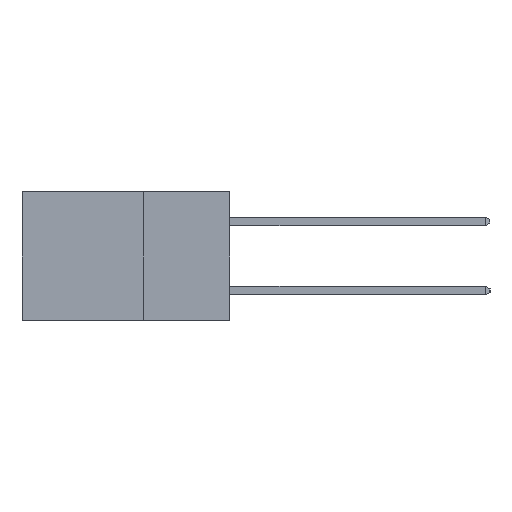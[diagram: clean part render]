
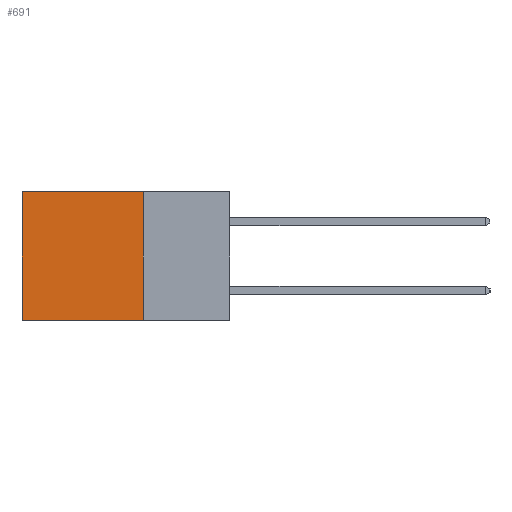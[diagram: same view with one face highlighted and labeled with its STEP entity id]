
A CAD part, left-side view. The second image highlights one B-rep face of the part: STEP entity #691.
In plain terms, the highlighted planar face has unit normal (-1, 0, 0).
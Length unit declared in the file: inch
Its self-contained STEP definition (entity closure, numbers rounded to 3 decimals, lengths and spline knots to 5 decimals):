
#233 = VECTOR ( 'NONE', #857, 39.37008 ) ;
#343 = DIRECTION ( 'NONE',  ( 0., 0., -1. ) ) ;
#485 = AXIS2_PLACEMENT_3D ( 'NONE', #15992, #3323, #12492 ) ;
#618 = ORIENTED_EDGE ( 'NONE', *, *, #6132, .F. ) ;
#691 = ADVANCED_FACE ( 'NONE', ( #9687 ), #2797, .F. ) ;
#857 = DIRECTION ( 'NONE',  ( 0., 1., 0. ) ) ;
#2797 = PLANE ( 'NONE',  #485 ) ;
#2810 = VERTEX_POINT ( 'NONE', #12886 ) ;
#3323 = DIRECTION ( 'NONE',  ( 1., 0., 0. ) ) ;
#3816 = EDGE_LOOP ( 'NONE', ( #7078, #16135, #618, #5748 ) ) ;
#4858 = DIRECTION ( 'NONE',  ( 0., 0., -1. ) ) ;
#4925 = VERTEX_POINT ( 'NONE', #6844 ) ;
#5748 = ORIENTED_EDGE ( 'NONE', *, *, #8540, .T. ) ;
#6132 = EDGE_CURVE ( 'NONE', #9060, #4925, #10364, .T. ) ;
#6844 = CARTESIAN_POINT ( 'NONE',  ( 0.2615, 0.25, -0.37 ) ) ;
#7078 = ORIENTED_EDGE ( 'NONE', *, *, #8276, .T. ) ;
#7464 = CARTESIAN_POINT ( 'NONE',  ( 0.2615, 0.25, -0.37 ) ) ;
#8150 = LINE ( 'NONE', #7464, #12602 ) ;
#8276 = EDGE_CURVE ( 'NONE', #2810, #11419, #8672, .T. ) ;
#8512 = CARTESIAN_POINT ( 'NONE',  ( 0.2615, 0.25, 0. ) ) ;
#8540 = EDGE_CURVE ( 'NONE', #9060, #2810, #15463, .T. ) ;
#8672 = LINE ( 'NONE', #15400, #12179 ) ;
#9060 = VERTEX_POINT ( 'NONE', #17175 ) ;
#9687 = FACE_OUTER_BOUND ( 'NONE', #3816, .T. ) ;
#10364 = LINE ( 'NONE', #18531, #17468 ) ;
#11419 = VERTEX_POINT ( 'NONE', #13099 ) ;
#12179 = VECTOR ( 'NONE', #4858, 39.37008 ) ;
#12492 = DIRECTION ( 'NONE',  ( 0., 0., -1. ) ) ;
#12602 = VECTOR ( 'NONE', #13458, 39.37008 ) ;
#12886 = CARTESIAN_POINT ( 'NONE',  ( 0.2615, 0.6, 0. ) ) ;
#13099 = CARTESIAN_POINT ( 'NONE',  ( 0.2615, 0.6, -0.37 ) ) ;
#13458 = DIRECTION ( 'NONE',  ( 0., 1., 0. ) ) ;
#14696 = EDGE_CURVE ( 'NONE', #4925, #11419, #8150, .T. ) ;
#15400 = CARTESIAN_POINT ( 'NONE',  ( 0.2615, 0.6, -0.37 ) ) ;
#15463 = LINE ( 'NONE', #8512, #233 ) ;
#15992 = CARTESIAN_POINT ( 'NONE',  ( 0.2615, 0.25, -0.37 ) ) ;
#16135 = ORIENTED_EDGE ( 'NONE', *, *, #14696, .F. ) ;
#17175 = CARTESIAN_POINT ( 'NONE',  ( 0.2615, 0.25, 0. ) ) ;
#17468 = VECTOR ( 'NONE', #343, 39.37008 ) ;
#18531 = CARTESIAN_POINT ( 'NONE',  ( 0.2615, 0.25, -0.37 ) ) ;
